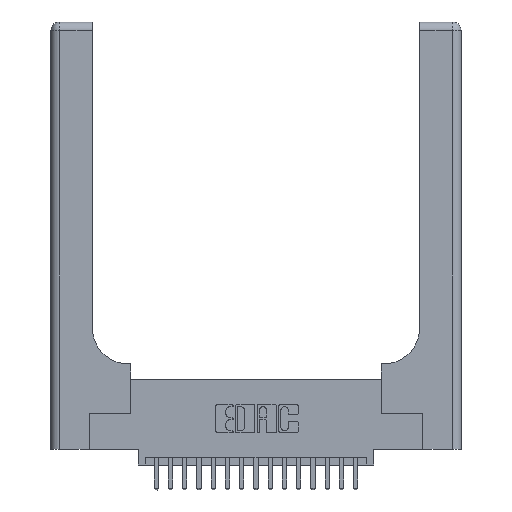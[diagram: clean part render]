
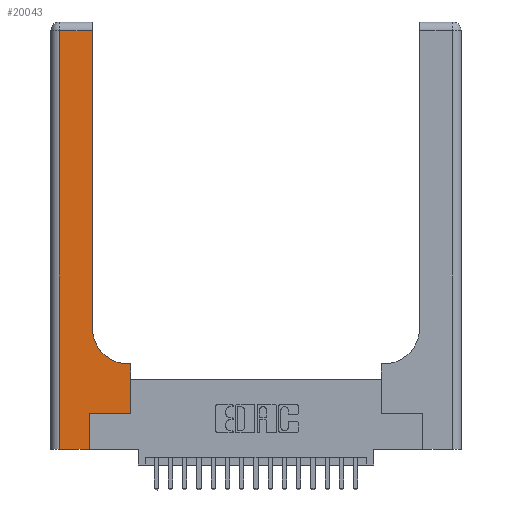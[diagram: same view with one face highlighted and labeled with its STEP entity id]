
A CAD part, top view. The second image highlights one B-rep face of the part: STEP entity #20043.
In plain terms, the highlighted planar face has unit normal (0, 0, 1).
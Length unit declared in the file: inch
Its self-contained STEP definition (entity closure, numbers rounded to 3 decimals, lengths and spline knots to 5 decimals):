
#60 = CARTESIAN_POINT ( 'NONE',  ( 0., 3., 0.37 ) ) ;
#216 = LINE ( 'NONE', #20664, #470 ) ;
#251 = LINE ( 'NONE', #5178, #6283 ) ;
#470 = VECTOR ( 'NONE', #4688, 39.37008 ) ;
#815 = ORIENTED_EDGE ( 'NONE', *, *, #2886, .T. ) ;
#1119 = ORIENTED_EDGE ( 'NONE', *, *, #4973, .T. ) ;
#1412 = VECTOR ( 'NONE', #5071, 39.37008 ) ;
#1566 = VERTEX_POINT ( 'NONE', #20419 ) ;
#1679 = VERTEX_POINT ( 'NONE', #6266 ) ;
#1720 = CARTESIAN_POINT ( 'NONE',  ( 0.5585, 0.25, 0.37 ) ) ;
#1973 = VECTOR ( 'NONE', #12983, 39.37008 ) ;
#2731 = EDGE_CURVE ( 'NONE', #3349, #14403, #216, .T. ) ;
#2825 = CARTESIAN_POINT ( 'NONE',  ( 0.5585, 0.25, 0.37 ) ) ;
#2886 = EDGE_CURVE ( 'NONE', #14403, #8144, #13834, .T. ) ;
#2926 = FACE_OUTER_BOUND ( 'NONE', #5550, .T. ) ;
#2996 = EDGE_CURVE ( 'NONE', #1566, #3349, #19870, .T. ) ;
#3349 = VERTEX_POINT ( 'NONE', #20568 ) ;
#3438 = DIRECTION ( 'NONE',  ( 0., 1., 0. ) ) ;
#3614 = CARTESIAN_POINT ( 'NONE',  ( 0.269, 0.25, 0.37 ) ) ;
#4014 = DIRECTION ( 'NONE',  ( 0., 0., -1. ) ) ;
#4481 = VECTOR ( 'NONE', #20040, 39.37008 ) ;
#4688 = DIRECTION ( 'NONE',  ( 1., 0., 0. ) ) ;
#4711 = DIRECTION ( 'NONE',  ( 0., 0., -1. ) ) ;
#4973 = EDGE_CURVE ( 'NONE', #9482, #1566, #7730, .T. ) ;
#5071 = DIRECTION ( 'NONE',  ( -1., 0., 0. ) ) ;
#5143 = VERTEX_POINT ( 'NONE', #9045 ) ;
#5178 = CARTESIAN_POINT ( 'NONE',  ( 0.269, 0.25, 0.37 ) ) ;
#5419 = EDGE_CURVE ( 'NONE', #1679, #15552, #16494, .T. ) ;
#5550 = EDGE_LOOP ( 'NONE', ( #14709, #1119, #13371, #9732, #815, #5609, #10589, #9404, #6606 ) ) ;
#5609 = ORIENTED_EDGE ( 'NONE', *, *, #7357, .T. ) ;
#6266 = CARTESIAN_POINT ( 'NONE',  ( 0.5585, 0.6, 0.37 ) ) ;
#6283 = VECTOR ( 'NONE', #19545, 39.37008 ) ;
#6530 = DIRECTION ( 'NONE',  ( -1., 0., 0. ) ) ;
#6606 = ORIENTED_EDGE ( 'NONE', *, *, #14041, .T. ) ;
#7357 = EDGE_CURVE ( 'NONE', #8144, #19953, #251, .T. ) ;
#7417 = VECTOR ( 'NONE', #6530, 39.37008 ) ;
#7730 = LINE ( 'NONE', #9834, #1412 ) ;
#7895 = PLANE ( 'NONE',  #20646 ) ;
#8144 = VERTEX_POINT ( 'NONE', #3614 ) ;
#8289 = VECTOR ( 'NONE', #14832, 39.37008 ) ;
#8847 = CARTESIAN_POINT ( 'NONE',  ( 0.5415, 0.85, 0.37 ) ) ;
#9045 = CARTESIAN_POINT ( 'NONE',  ( 0.2915, 0.85, 0.37 ) ) ;
#9404 = ORIENTED_EDGE ( 'NONE', *, *, #5419, .T. ) ;
#9482 = VERTEX_POINT ( 'NONE', #18121 ) ;
#9732 = ORIENTED_EDGE ( 'NONE', *, *, #2731, .T. ) ;
#9834 = CARTESIAN_POINT ( 'NONE',  ( 0., 2.94, 0.37 ) ) ;
#10006 = LINE ( 'NONE', #1720, #1973 ) ;
#10207 = CARTESIAN_POINT ( 'NONE',  ( 0.5415, 0.6, 0.37 ) ) ;
#10554 = VECTOR ( 'NONE', #3438, 39.37008 ) ;
#10589 = ORIENTED_EDGE ( 'NONE', *, *, #19513, .T. ) ;
#12070 = LINE ( 'NONE', #13069, #10554 ) ;
#12983 = DIRECTION ( 'NONE',  ( 0., 1., 0. ) ) ;
#13069 = CARTESIAN_POINT ( 'NONE',  ( 0.2915, 3., 0.37 ) ) ;
#13142 = CARTESIAN_POINT ( 'NONE',  ( 0.269, 0., 0.37 ) ) ;
#13302 = DIRECTION ( 'NONE',  ( 1., 0., 0. ) ) ;
#13371 = ORIENTED_EDGE ( 'NONE', *, *, #2996, .T. ) ;
#13432 = CARTESIAN_POINT ( 'NONE',  ( 0.06, 3., 0.37 ) ) ;
#13834 = LINE ( 'NONE', #13142, #8289 ) ;
#14041 = EDGE_CURVE ( 'NONE', #15552, #5143, #20497, .T. ) ;
#14403 = VERTEX_POINT ( 'NONE', #17308 ) ;
#14708 = CARTESIAN_POINT ( 'NONE',  ( 0.2915, 0.6, 0.37 ) ) ;
#14709 = ORIENTED_EDGE ( 'NONE', *, *, #18815, .T. ) ;
#14832 = DIRECTION ( 'NONE',  ( 0., 1., 0. ) ) ;
#15552 = VERTEX_POINT ( 'NONE', #10207 ) ;
#16277 = AXIS2_PLACEMENT_3D ( 'NONE', #8847, #4014, #13302 ) ;
#16494 = LINE ( 'NONE', #14708, #7417 ) ;
#17308 = CARTESIAN_POINT ( 'NONE',  ( 0.269, 0., 0.37 ) ) ;
#18121 = CARTESIAN_POINT ( 'NONE',  ( 0.2915, 2.94, 0.37 ) ) ;
#18815 = EDGE_CURVE ( 'NONE', #5143, #9482, #12070, .T. ) ;
#19367 = DIRECTION ( 'NONE',  ( -1., 0., 0. ) ) ;
#19513 = EDGE_CURVE ( 'NONE', #19953, #1679, #10006, .T. ) ;
#19545 = DIRECTION ( 'NONE',  ( 1., 0., 0. ) ) ;
#19870 = LINE ( 'NONE', #13432, #4481 ) ;
#19953 = VERTEX_POINT ( 'NONE', #2825 ) ;
#20040 = DIRECTION ( 'NONE',  ( 0., -1., 0. ) ) ;
#20043 = ADVANCED_FACE ( 'NONE', ( #2926 ), #7895, .F. ) ;
#20419 = CARTESIAN_POINT ( 'NONE',  ( 0.06, 2.94, 0.37 ) ) ;
#20497 = CIRCLE ( 'NONE', #16277, 0.25 ) ;
#20568 = CARTESIAN_POINT ( 'NONE',  ( 0.06, 0., 0.37 ) ) ;
#20646 = AXIS2_PLACEMENT_3D ( 'NONE', #60, #4711, #19367 ) ;
#20664 = CARTESIAN_POINT ( 'NONE',  ( 0., 0., 0.37 ) ) ;
